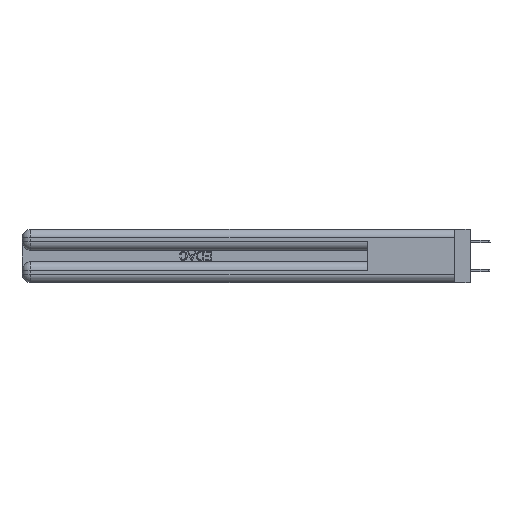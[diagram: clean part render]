
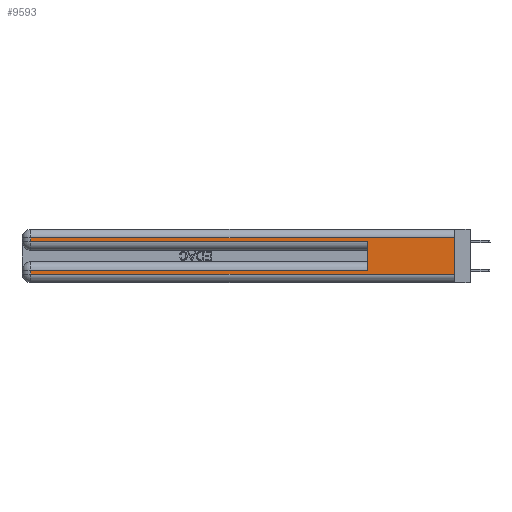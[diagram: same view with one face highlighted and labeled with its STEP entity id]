
A CAD part, left-side view. The second image highlights one B-rep face of the part: STEP entity #9593.
In plain terms, the highlighted planar face has unit normal (-1, 0, 0).
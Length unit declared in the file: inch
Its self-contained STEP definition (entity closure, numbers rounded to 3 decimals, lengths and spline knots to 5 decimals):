
#302 = VERTEX_POINT ( 'NONE', #33021 ) ;
#937 = LINE ( 'NONE', #24137, #41867 ) ;
#1845 = FACE_OUTER_BOUND ( 'NONE', #31956, .T. ) ;
#4934 = DIRECTION ( 'NONE',  ( 0., 0., -1. ) ) ;
#6037 = VERTEX_POINT ( 'NONE', #38518 ) ;
#6290 = ORIENTED_EDGE ( 'NONE', *, *, #36523, .T. ) ;
#6774 = DIRECTION ( 'NONE',  ( 0., 0., -1. ) ) ;
#7462 = VECTOR ( 'NONE', #35600, 39.37008 ) ;
#8137 = EDGE_CURVE ( 'NONE', #15984, #41447, #16271, .T. ) ;
#8889 = ORIENTED_EDGE ( 'NONE', *, *, #8137, .T. ) ;
#8913 = CARTESIAN_POINT ( 'NONE',  ( 0., 0., 0.06 ) ) ;
#9593 = ADVANCED_FACE ( 'NONE', ( #1845 ), #28783, .F. ) ;
#10284 = ORIENTED_EDGE ( 'NONE', *, *, #34178, .T. ) ;
#10770 = ORIENTED_EDGE ( 'NONE', *, *, #25571, .F. ) ;
#11106 = ORIENTED_EDGE ( 'NONE', *, *, #19307, .T. ) ;
#12029 = DIRECTION ( 'NONE',  ( 0., -1., 0. ) ) ;
#12211 = DIRECTION ( 'NONE',  ( 0., 0., -1. ) ) ;
#14376 = CARTESIAN_POINT ( 'NONE',  ( 0., 0., 0.085 ) ) ;
#14653 = VECTOR ( 'NONE', #17482, 39.37008 ) ;
#15260 = LINE ( 'NONE', #29209, #21041 ) ;
#15984 = VERTEX_POINT ( 'NONE', #40302 ) ;
#16271 = LINE ( 'NONE', #23568, #30841 ) ;
#17482 = DIRECTION ( 'NONE',  ( 0., 1., 0. ) ) ;
#18847 = VERTEX_POINT ( 'NONE', #39923 ) ;
#19307 = EDGE_CURVE ( 'NONE', #6037, #15984, #34551, .T. ) ;
#20186 = EDGE_CURVE ( 'NONE', #26361, #32460, #39146, .T. ) ;
#20540 = DIRECTION ( 'NONE',  ( 0., 0., -1. ) ) ;
#20575 = LINE ( 'NONE', #14376, #14653 ) ;
#21041 = VECTOR ( 'NONE', #12211, 39.37008 ) ;
#23047 = CARTESIAN_POINT ( 'NONE',  ( 0., 0., 0.06 ) ) ;
#23568 = CARTESIAN_POINT ( 'NONE',  ( 0., 2.94, 0.37 ) ) ;
#23971 = DIRECTION ( 'NONE',  ( 0., 1., 0. ) ) ;
#24137 = CARTESIAN_POINT ( 'NONE',  ( 0., 0.6, 0.145 ) ) ;
#24539 = EDGE_CURVE ( 'NONE', #6037, #32460, #33393, .T. ) ;
#25571 = EDGE_CURVE ( 'NONE', #302, #18847, #937, .T. ) ;
#26361 = VERTEX_POINT ( 'NONE', #40009 ) ;
#27717 = CARTESIAN_POINT ( 'NONE',  ( 0., 0., 0.31 ) ) ;
#28554 = LINE ( 'NONE', #42849, #7462 ) ;
#28783 = PLANE ( 'NONE',  #35184 ) ;
#29209 = CARTESIAN_POINT ( 'NONE',  ( 0., 2.94, 0.37 ) ) ;
#30067 = CARTESIAN_POINT ( 'NONE',  ( 0., 0., 0.37 ) ) ;
#30434 = VERTEX_POINT ( 'NONE', #36619 ) ;
#30841 = VECTOR ( 'NONE', #6774, 39.37008 ) ;
#31412 = EDGE_CURVE ( 'NONE', #41447, #18847, #28554, .T. ) ;
#31597 = ORIENTED_EDGE ( 'NONE', *, *, #20186, .T. ) ;
#31956 = EDGE_LOOP ( 'NONE', ( #34064, #11106, #8889, #40647, #10770, #10284, #6290, #31597 ) ) ;
#32460 = VERTEX_POINT ( 'NONE', #23047 ) ;
#32943 = CARTESIAN_POINT ( 'NONE',  ( 0., 2.94, 0.285 ) ) ;
#33021 = CARTESIAN_POINT ( 'NONE',  ( 0., 0.6, 0.085 ) ) ;
#33393 = LINE ( 'NONE', #30067, #34068 ) ;
#34064 = ORIENTED_EDGE ( 'NONE', *, *, #24539, .F. ) ;
#34068 = VECTOR ( 'NONE', #20540, 39.37008 ) ;
#34178 = EDGE_CURVE ( 'NONE', #302, #30434, #20575, .T. ) ;
#34551 = LINE ( 'NONE', #27717, #37411 ) ;
#34964 = CARTESIAN_POINT ( 'NONE',  ( 0., 0., 0.37 ) ) ;
#35184 = AXIS2_PLACEMENT_3D ( 'NONE', #34964, #38686, #4934 ) ;
#35600 = DIRECTION ( 'NONE',  ( 0., -1., 0. ) ) ;
#36523 = EDGE_CURVE ( 'NONE', #30434, #26361, #15260, .T. ) ;
#36619 = CARTESIAN_POINT ( 'NONE',  ( 0., 2.94, 0.085 ) ) ;
#36766 = VECTOR ( 'NONE', #12029, 39.37008 ) ;
#37411 = VECTOR ( 'NONE', #23971, 39.37008 ) ;
#38518 = CARTESIAN_POINT ( 'NONE',  ( 0., 0., 0.31 ) ) ;
#38686 = DIRECTION ( 'NONE',  ( 1., 0., 0. ) ) ;
#39146 = LINE ( 'NONE', #8913, #36766 ) ;
#39923 = CARTESIAN_POINT ( 'NONE',  ( 0., 0.6, 0.285 ) ) ;
#40009 = CARTESIAN_POINT ( 'NONE',  ( 0., 2.94, 0.06 ) ) ;
#40302 = CARTESIAN_POINT ( 'NONE',  ( 0., 2.94, 0.31 ) ) ;
#40647 = ORIENTED_EDGE ( 'NONE', *, *, #31412, .T. ) ;
#41447 = VERTEX_POINT ( 'NONE', #32943 ) ;
#41758 = DIRECTION ( 'NONE',  ( 0., 0., 1. ) ) ;
#41867 = VECTOR ( 'NONE', #41758, 39.37008 ) ;
#42849 = CARTESIAN_POINT ( 'NONE',  ( 0., 0., 0.285 ) ) ;
